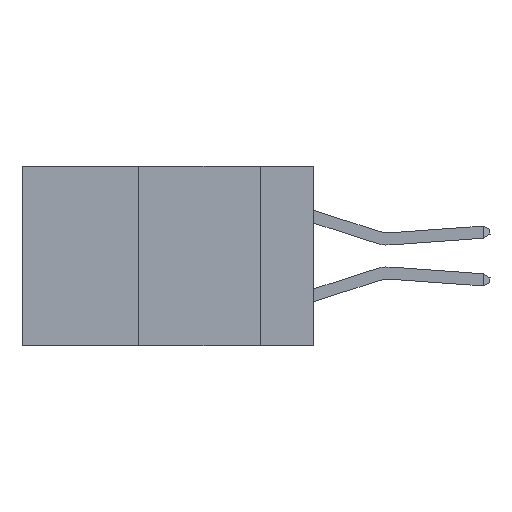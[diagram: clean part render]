
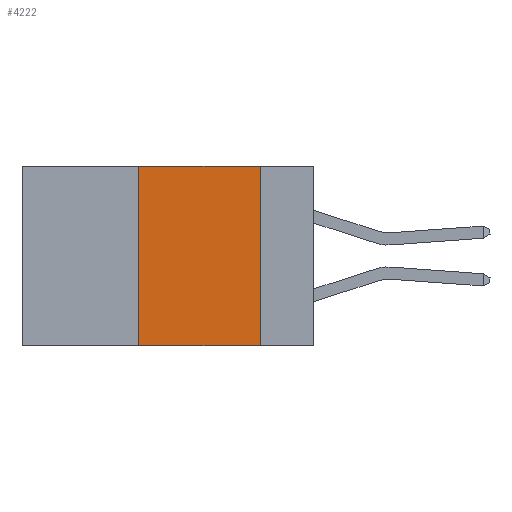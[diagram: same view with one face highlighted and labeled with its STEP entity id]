
A CAD part, left-side view. The second image highlights one B-rep face of the part: STEP entity #4222.
In plain terms, the highlighted planar face has unit normal (-1, 0, 0).
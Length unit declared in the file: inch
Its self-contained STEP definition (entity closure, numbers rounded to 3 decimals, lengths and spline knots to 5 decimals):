
#959 = EDGE_CURVE ( 'NONE', #10168, #6418, #6991, .T. ) ;
#1030 = PLANE ( 'NONE',  #2216 ) ;
#1336 = CARTESIAN_POINT ( 'NONE',  ( 0., 0.11, -0.37 ) ) ;
#1471 = VECTOR ( 'NONE', #12845, 39.37008 ) ;
#1564 = VECTOR ( 'NONE', #11993, 39.37008 ) ;
#2216 = AXIS2_PLACEMENT_3D ( 'NONE', #5029, #10928, #12047 ) ;
#2870 = CARTESIAN_POINT ( 'NONE',  ( 0., 0.11, 0. ) ) ;
#3094 = ORIENTED_EDGE ( 'NONE', *, *, #7324, .T. ) ;
#3641 = CARTESIAN_POINT ( 'NONE',  ( 0., 0.36, 0. ) ) ;
#3672 = EDGE_CURVE ( 'NONE', #6418, #5355, #4504, .T. ) ;
#3865 = FACE_OUTER_BOUND ( 'NONE', #7470, .T. ) ;
#3956 = LINE ( 'NONE', #8728, #1471 ) ;
#4222 = ADVANCED_FACE ( 'NONE', ( #3865 ), #1030, .F. ) ;
#4294 = DIRECTION ( 'NONE',  ( 0., 0., 1. ) ) ;
#4504 = LINE ( 'NONE', #6073, #1564 ) ;
#4995 = CARTESIAN_POINT ( 'NONE',  ( 0., 0.36, -0.37 ) ) ;
#5029 = CARTESIAN_POINT ( 'NONE',  ( 0., 0.6, 0. ) ) ;
#5355 = VERTEX_POINT ( 'NONE', #2870 ) ;
#5726 = VERTEX_POINT ( 'NONE', #1336 ) ;
#5805 = ORIENTED_EDGE ( 'NONE', *, *, #959, .F. ) ;
#6073 = CARTESIAN_POINT ( 'NONE',  ( 0., 0.6, 0. ) ) ;
#6418 = VERTEX_POINT ( 'NONE', #3641 ) ;
#6991 = LINE ( 'NONE', #12388, #7308 ) ;
#7308 = VECTOR ( 'NONE', #4294, 39.37008 ) ;
#7324 = EDGE_CURVE ( 'NONE', #10168, #5726, #3956, .T. ) ;
#7440 = VECTOR ( 'NONE', #12347, 39.37008 ) ;
#7470 = EDGE_LOOP ( 'NONE', ( #9259, #12291, #5805, #3094 ) ) ;
#7744 = LINE ( 'NONE', #11335, #7440 ) ;
#8728 = CARTESIAN_POINT ( 'NONE',  ( 0., 0.6, -0.37 ) ) ;
#9259 = ORIENTED_EDGE ( 'NONE', *, *, #12829, .F. ) ;
#10168 = VERTEX_POINT ( 'NONE', #4995 ) ;
#10928 = DIRECTION ( 'NONE',  ( 1., 0., 0. ) ) ;
#11335 = CARTESIAN_POINT ( 'NONE',  ( 0., 0.11, 0. ) ) ;
#11993 = DIRECTION ( 'NONE',  ( 0., -1., 0. ) ) ;
#12047 = DIRECTION ( 'NONE',  ( 0., 0., -1. ) ) ;
#12291 = ORIENTED_EDGE ( 'NONE', *, *, #3672, .F. ) ;
#12347 = DIRECTION ( 'NONE',  ( 0., 0., -1. ) ) ;
#12388 = CARTESIAN_POINT ( 'NONE',  ( 0., 0.36, 0. ) ) ;
#12829 = EDGE_CURVE ( 'NONE', #5355, #5726, #7744, .T. ) ;
#12845 = DIRECTION ( 'NONE',  ( 0., -1., 0. ) ) ;
